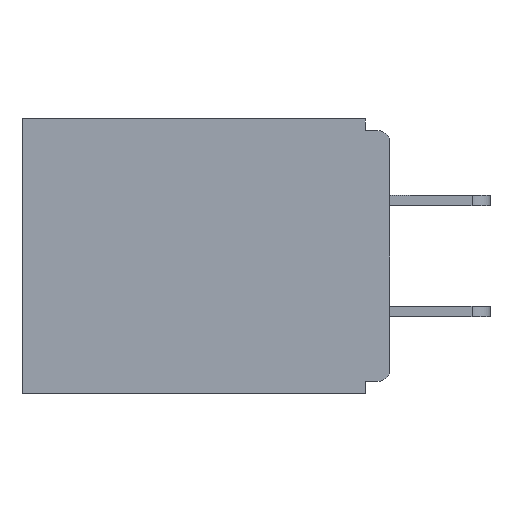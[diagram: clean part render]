
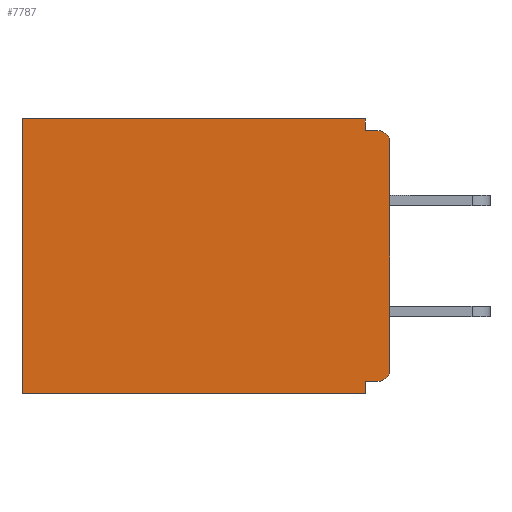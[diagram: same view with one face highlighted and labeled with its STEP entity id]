
A CAD part, left-side view. The second image highlights one B-rep face of the part: STEP entity #7787.
In plain terms, the highlighted planar face has unit normal (-1, 0, 0).
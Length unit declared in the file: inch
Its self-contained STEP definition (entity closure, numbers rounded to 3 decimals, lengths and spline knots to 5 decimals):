
#380 = VERTEX_POINT ( 'NONE', #20416 ) ;
#1432 = LINE ( 'NONE', #8326, #22780 ) ;
#1541 = VERTEX_POINT ( 'NONE', #18387 ) ;
#1731 = EDGE_CURVE ( 'NONE', #21455, #1541, #20592, .T. ) ;
#1879 = ORIENTED_EDGE ( 'NONE', *, *, #21925, .F. ) ;
#2126 = DIRECTION ( 'NONE',  ( -1., 0., 0. ) ) ;
#2265 = CARTESIAN_POINT ( 'NONE',  ( 0.298, 0., -0.015 ) ) ;
#2851 = VERTEX_POINT ( 'NONE', #16257 ) ;
#3545 = DIRECTION ( 'NONE',  ( 0., 0., -1. ) ) ;
#3659 = FACE_OUTER_BOUND ( 'NONE', #13407, .T. ) ;
#3710 = LINE ( 'NONE', #21534, #22866 ) ;
#4436 = DIRECTION ( 'NONE',  ( 0., 0., -1. ) ) ;
#4505 = ORIENTED_EDGE ( 'NONE', *, *, #19148, .T. ) ;
#5128 = CARTESIAN_POINT ( 'NONE',  ( 0.298, 0.46, 0. ) ) ;
#5440 = EDGE_CURVE ( 'NONE', #17425, #2851, #20421, .T. ) ;
#5441 = LINE ( 'NONE', #19206, #15161 ) ;
#5459 = DIRECTION ( 'NONE',  ( 0., 0., -1. ) ) ;
#5646 = ORIENTED_EDGE ( 'NONE', *, *, #15218, .F. ) ;
#5886 = DIRECTION ( 'NONE',  ( 0., 1., 0. ) ) ;
#5981 = VERTEX_POINT ( 'NONE', #22834 ) ;
#6142 = EDGE_CURVE ( 'NONE', #380, #2851, #22292, .T. ) ;
#6792 = EDGE_CURVE ( 'NONE', #13207, #1541, #3710, .T. ) ;
#6947 = CARTESIAN_POINT ( 'NONE',  ( 0.298, 0., 0. ) ) ;
#7433 = DIRECTION ( 'NONE',  ( 0., 0., -1. ) ) ;
#7511 = CARTESIAN_POINT ( 'NONE',  ( 0.298, 0.031, -0.343 ) ) ;
#7621 = AXIS2_PLACEMENT_3D ( 'NONE', #21439, #15959, #14104 ) ;
#7622 = ORIENTED_EDGE ( 'NONE', *, *, #8337, .T. ) ;
#7682 = AXIS2_PLACEMENT_3D ( 'NONE', #12730, #2126, #7433 ) ;
#7787 = ADVANCED_FACE ( 'NONE', ( #3659 ), #12481, .F. ) ;
#8326 = CARTESIAN_POINT ( 'NONE',  ( 0.298, 0., -0.328 ) ) ;
#8337 = EDGE_CURVE ( 'NONE', #5981, #21455, #8862, .T. ) ;
#8393 = DIRECTION ( 'NONE',  ( 0., 1., 0. ) ) ;
#8862 = LINE ( 'NONE', #9014, #22204 ) ;
#9014 = CARTESIAN_POINT ( 'NONE',  ( 0.298, 0., 0. ) ) ;
#9079 = EDGE_CURVE ( 'NONE', #12528, #13207, #17791, .T. ) ;
#9264 = AXIS2_PLACEMENT_3D ( 'NONE', #6947, #10574, #3545 ) ;
#9749 = ORIENTED_EDGE ( 'NONE', *, *, #9079, .F. ) ;
#10179 = ORIENTED_EDGE ( 'NONE', *, *, #1731, .T. ) ;
#10565 = LINE ( 'NONE', #16336, #18963 ) ;
#10574 = DIRECTION ( 'NONE',  ( 1., 0., 0. ) ) ;
#11209 = ORIENTED_EDGE ( 'NONE', *, *, #21048, .F. ) ;
#11386 = VECTOR ( 'NONE', #4436, 39.37008 ) ;
#12015 = CARTESIAN_POINT ( 'NONE',  ( 0.298, 0., -0.313 ) ) ;
#12481 = PLANE ( 'NONE',  #9264 ) ;
#12528 = VERTEX_POINT ( 'NONE', #22686 ) ;
#12730 = CARTESIAN_POINT ( 'NONE',  ( 0.298, 0.015, -0.313 ) ) ;
#13207 = VERTEX_POINT ( 'NONE', #21251 ) ;
#13378 = ORIENTED_EDGE ( 'NONE', *, *, #6792, .F. ) ;
#13407 = EDGE_LOOP ( 'NONE', ( #19239, #19558, #5646, #7622, #10179, #13378, #9749, #1879, #4505, #11209 ) ) ;
#13633 = DIRECTION ( 'NONE',  ( 0., 1., 0. ) ) ;
#14104 = DIRECTION ( 'NONE',  ( 0., 0., -1. ) ) ;
#14145 = VERTEX_POINT ( 'NONE', #22429 ) ;
#14606 = CIRCLE ( 'NONE', #7682, 0.015 ) ;
#14923 = DIRECTION ( 'NONE',  ( 0., 0., -1. ) ) ;
#15161 = VECTOR ( 'NONE', #17264, 39.37008 ) ;
#15218 = EDGE_CURVE ( 'NONE', #5981, #17425, #5441, .T. ) ;
#15841 = CARTESIAN_POINT ( 'NONE',  ( 0.298, 0.031, -0.015 ) ) ;
#15959 = DIRECTION ( 'NONE',  ( -1., 0., 0. ) ) ;
#16119 = VECTOR ( 'NONE', #14923, 39.37008 ) ;
#16257 = CARTESIAN_POINT ( 'NONE',  ( 0.298, 0.015, -0.015 ) ) ;
#16336 = CARTESIAN_POINT ( 'NONE',  ( 0.298, 0., 0. ) ) ;
#17264 = DIRECTION ( 'NONE',  ( 0., 0., -1. ) ) ;
#17425 = VERTEX_POINT ( 'NONE', #15841 ) ;
#17791 = LINE ( 'NONE', #7511, #16119 ) ;
#18387 = CARTESIAN_POINT ( 'NONE',  ( 0.298, 0.46, -0.343 ) ) ;
#18499 = DIRECTION ( 'NONE',  ( 0., -1., 0. ) ) ;
#18508 = VECTOR ( 'NONE', #18499, 39.37008 ) ;
#18963 = VECTOR ( 'NONE', #5459, 39.37008 ) ;
#19148 = EDGE_CURVE ( 'NONE', #14145, #19362, #14606, .T. ) ;
#19206 = CARTESIAN_POINT ( 'NONE',  ( 0.298, 0.031, -0.343 ) ) ;
#19239 = ORIENTED_EDGE ( 'NONE', *, *, #6142, .T. ) ;
#19362 = VERTEX_POINT ( 'NONE', #12015 ) ;
#19558 = ORIENTED_EDGE ( 'NONE', *, *, #5440, .F. ) ;
#20416 = CARTESIAN_POINT ( 'NONE',  ( 0.298, 0., -0.03 ) ) ;
#20421 = LINE ( 'NONE', #2265, #18508 ) ;
#20592 = LINE ( 'NONE', #22112, #11386 ) ;
#21048 = EDGE_CURVE ( 'NONE', #380, #19362, #10565, .T. ) ;
#21251 = CARTESIAN_POINT ( 'NONE',  ( 0.298, 0.031, -0.343 ) ) ;
#21439 = CARTESIAN_POINT ( 'NONE',  ( 0.298, 0.015, -0.03 ) ) ;
#21455 = VERTEX_POINT ( 'NONE', #5128 ) ;
#21534 = CARTESIAN_POINT ( 'NONE',  ( 0.298, 0., -0.343 ) ) ;
#21925 = EDGE_CURVE ( 'NONE', #14145, #12528, #1432, .T. ) ;
#22112 = CARTESIAN_POINT ( 'NONE',  ( 0.298, 0.46, 0. ) ) ;
#22204 = VECTOR ( 'NONE', #8393, 39.37008 ) ;
#22292 = CIRCLE ( 'NONE', #7621, 0.015 ) ;
#22429 = CARTESIAN_POINT ( 'NONE',  ( 0.298, 0.015, -0.328 ) ) ;
#22686 = CARTESIAN_POINT ( 'NONE',  ( 0.298, 0.031, -0.328 ) ) ;
#22780 = VECTOR ( 'NONE', #13633, 39.37008 ) ;
#22834 = CARTESIAN_POINT ( 'NONE',  ( 0.298, 0.031, 0. ) ) ;
#22866 = VECTOR ( 'NONE', #5886, 39.37008 ) ;
